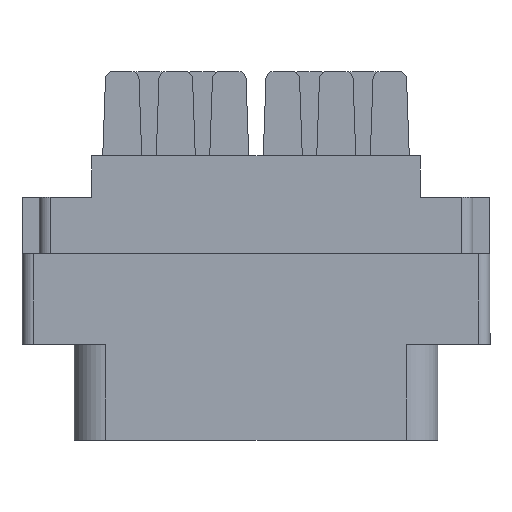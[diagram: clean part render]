
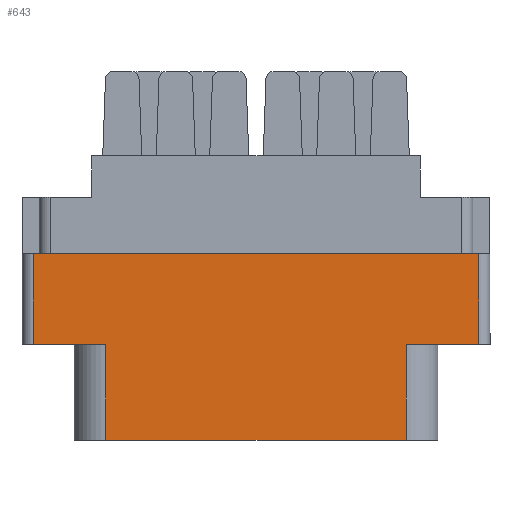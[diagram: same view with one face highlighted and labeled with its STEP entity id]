
A CAD part, front view. The second image highlights one B-rep face of the part: STEP entity #643.
In plain terms, the highlighted planar face has unit normal (0, -1, 0).
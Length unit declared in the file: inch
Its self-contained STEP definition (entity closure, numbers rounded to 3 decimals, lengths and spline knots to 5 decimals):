
#118 = ORIENTED_EDGE ( 'NONE', *, *, #16848, .T. ) ;
#634 = VECTOR ( 'NONE', #19641, 39.37008 ) ;
#643 = ADVANCED_FACE ( 'NONE', ( #1916 ), #3736, .T. ) ;
#826 = VERTEX_POINT ( 'NONE', #21865 ) ;
#944 = VECTOR ( 'NONE', #17431, 39.37008 ) ;
#1502 = LINE ( 'NONE', #3546, #18706 ) ;
#1621 = LINE ( 'NONE', #19760, #13422 ) ;
#1916 = FACE_OUTER_BOUND ( 'NONE', #17159, .T. ) ;
#1919 = EDGE_CURVE ( 'NONE', #826, #10894, #1502, .T. ) ;
#3498 = CARTESIAN_POINT ( 'NONE',  ( -0.656, -0.343, -0.798 ) ) ;
#3546 = CARTESIAN_POINT ( 'NONE',  ( -0.656, -0.343, -0.798 ) ) ;
#3736 = PLANE ( 'NONE',  #9099 ) ;
#3849 = DIRECTION ( 'NONE',  ( 0., -1., 0. ) ) ;
#4206 = EDGE_CURVE ( 'NONE', #11162, #6412, #10455, .T. ) ;
#4369 = LINE ( 'NONE', #10063, #944 ) ;
#5472 = DIRECTION ( 'NONE',  ( 1., 0., 0. ) ) ;
#6239 = CARTESIAN_POINT ( 'NONE',  ( -0.42052, -0.343, -0.798 ) ) ;
#6412 = VERTEX_POINT ( 'NONE', #19405 ) ;
#6595 = EDGE_CURVE ( 'NONE', #10894, #18510, #20322, .T. ) ;
#7022 = ORIENTED_EDGE ( 'NONE', *, *, #7838, .T. ) ;
#7710 = LINE ( 'NONE', #21759, #10702 ) ;
#7786 = CARTESIAN_POINT ( 'NONE',  ( 0.42052, -0.343, -0.529 ) ) ;
#7838 = EDGE_CURVE ( 'NONE', #17756, #11162, #1621, .T. ) ;
#8170 = LINE ( 'NONE', #6239, #16246 ) ;
#8218 = ORIENTED_EDGE ( 'NONE', *, *, #6595, .T. ) ;
#8326 = VECTOR ( 'NONE', #21262, 39.37008 ) ;
#8768 = DIRECTION ( 'NONE',  ( 0., 0., -1. ) ) ;
#8801 = LINE ( 'NONE', #16181, #8326 ) ;
#9099 = AXIS2_PLACEMENT_3D ( 'NONE', #3498, #3849, #18594 ) ;
#10063 = CARTESIAN_POINT ( 'NONE',  ( 0.624, -0.343, -0.798 ) ) ;
#10226 = ORIENTED_EDGE ( 'NONE', *, *, #4206, .T. ) ;
#10455 = LINE ( 'NONE', #14200, #634 ) ;
#10457 = DIRECTION ( 'NONE',  ( 0., 0., 1. ) ) ;
#10702 = VECTOR ( 'NONE', #19820, 39.37008 ) ;
#10894 = VERTEX_POINT ( 'NONE', #12637 ) ;
#11162 = VERTEX_POINT ( 'NONE', #11538 ) ;
#11371 = CARTESIAN_POINT ( 'NONE',  ( 0.624, -0.343, -0.529 ) ) ;
#11538 = CARTESIAN_POINT ( 'NONE',  ( -0.624, -0.343, -0.529 ) ) ;
#11730 = CARTESIAN_POINT ( 'NONE',  ( -0.624, -0.343, -0.274 ) ) ;
#11925 = DIRECTION ( 'NONE',  ( 0., 0., -1. ) ) ;
#12637 = CARTESIAN_POINT ( 'NONE',  ( 0.42052, -0.343, -0.798 ) ) ;
#13422 = VECTOR ( 'NONE', #8768, 39.37008 ) ;
#14200 = CARTESIAN_POINT ( 'NONE',  ( 0., -0.343, -0.529 ) ) ;
#14790 = ORIENTED_EDGE ( 'NONE', *, *, #20120, .T. ) ;
#15325 = VECTOR ( 'NONE', #10457, 39.37008 ) ;
#16181 = CARTESIAN_POINT ( 'NONE',  ( 0., -0.343, -0.529 ) ) ;
#16246 = VECTOR ( 'NONE', #11925, 39.37008 ) ;
#16692 = CARTESIAN_POINT ( 'NONE',  ( 0.42052, -0.343, -0.529 ) ) ;
#16848 = EDGE_CURVE ( 'NONE', #6412, #826, #8170, .T. ) ;
#17159 = EDGE_LOOP ( 'NONE', ( #18369, #7022, #10226, #118, #21657, #8218, #21579, #14790 ) ) ;
#17431 = DIRECTION ( 'NONE',  ( 0., 0., 1. ) ) ;
#17756 = VERTEX_POINT ( 'NONE', #11730 ) ;
#18369 = ORIENTED_EDGE ( 'NONE', *, *, #22773, .F. ) ;
#18510 = VERTEX_POINT ( 'NONE', #7786 ) ;
#18594 = DIRECTION ( 'NONE',  ( 0., 0., -1. ) ) ;
#18706 = VECTOR ( 'NONE', #5472, 39.37008 ) ;
#18958 = VERTEX_POINT ( 'NONE', #11371 ) ;
#19405 = CARTESIAN_POINT ( 'NONE',  ( -0.42052, -0.343, -0.529 ) ) ;
#19641 = DIRECTION ( 'NONE',  ( 1., 0., 0. ) ) ;
#19760 = CARTESIAN_POINT ( 'NONE',  ( -0.624, -0.343, -0.798 ) ) ;
#19820 = DIRECTION ( 'NONE',  ( 1., 0., 0. ) ) ;
#20004 = VERTEX_POINT ( 'NONE', #20200 ) ;
#20120 = EDGE_CURVE ( 'NONE', #18958, #20004, #4369, .T. ) ;
#20200 = CARTESIAN_POINT ( 'NONE',  ( 0.624, -0.343, -0.274 ) ) ;
#20322 = LINE ( 'NONE', #16692, #15325 ) ;
#21262 = DIRECTION ( 'NONE',  ( -1., 0., 0. ) ) ;
#21392 = EDGE_CURVE ( 'NONE', #18958, #18510, #8801, .T. ) ;
#21579 = ORIENTED_EDGE ( 'NONE', *, *, #21392, .F. ) ;
#21657 = ORIENTED_EDGE ( 'NONE', *, *, #1919, .T. ) ;
#21759 = CARTESIAN_POINT ( 'NONE',  ( 0., -0.343, -0.274 ) ) ;
#21865 = CARTESIAN_POINT ( 'NONE',  ( -0.42052, -0.343, -0.798 ) ) ;
#22773 = EDGE_CURVE ( 'NONE', #17756, #20004, #7710, .T. ) ;
